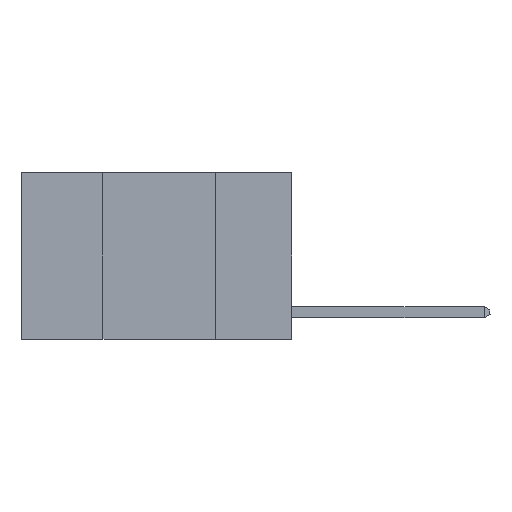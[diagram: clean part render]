
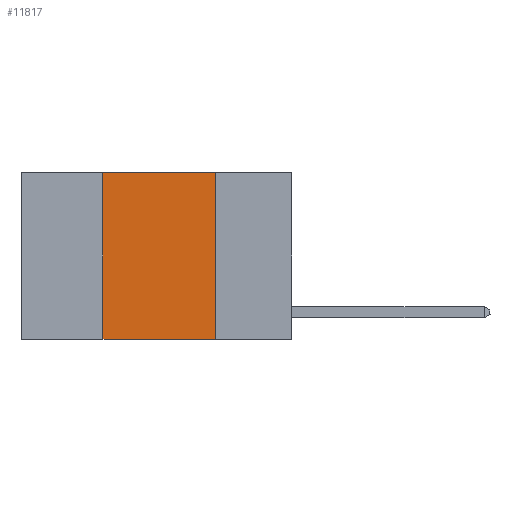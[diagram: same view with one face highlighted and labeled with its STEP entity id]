
A CAD part, left-side view. The second image highlights one B-rep face of the part: STEP entity #11817.
In plain terms, the highlighted planar face has unit normal (-1, 0, 0).
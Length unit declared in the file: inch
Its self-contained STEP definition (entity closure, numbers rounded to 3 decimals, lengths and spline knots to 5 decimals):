
#65 = VERTEX_POINT ( 'NONE', #8955 ) ;
#535 = LINE ( 'NONE', #18428, #4495 ) ;
#1374 = CARTESIAN_POINT ( 'NONE',  ( 0., 0.17, 0. ) ) ;
#2116 = EDGE_CURVE ( 'NONE', #18830, #6971, #5020, .T. ) ;
#3142 = DIRECTION ( 'NONE',  ( 0., 0., -1. ) ) ;
#4383 = EDGE_LOOP ( 'NONE', ( #15829, #8813, #13044, #15683 ) ) ;
#4392 = VECTOR ( 'NONE', #5676, 39.37008 ) ;
#4495 = VECTOR ( 'NONE', #13260, 39.37008 ) ;
#4566 = EDGE_CURVE ( 'NONE', #11226, #18830, #535, .T. ) ;
#4675 = AXIS2_PLACEMENT_3D ( 'NONE', #7570, #9560, #3142 ) ;
#5020 = LINE ( 'NONE', #12920, #7980 ) ;
#5676 = DIRECTION ( 'NONE',  ( 0., 0., -1. ) ) ;
#5678 = FACE_OUTER_BOUND ( 'NONE', #4383, .T. ) ;
#5888 = CARTESIAN_POINT ( 'NONE',  ( 0., 0.42, 0. ) ) ;
#6067 = VECTOR ( 'NONE', #16957, 39.37008 ) ;
#6500 = EDGE_CURVE ( 'NONE', #11226, #65, #10536, .T. ) ;
#6971 = VERTEX_POINT ( 'NONE', #1374 ) ;
#7246 = LINE ( 'NONE', #14931, #4392 ) ;
#7570 = CARTESIAN_POINT ( 'NONE',  ( 0., 0.6, 0. ) ) ;
#7980 = VECTOR ( 'NONE', #9772, 39.37008 ) ;
#8813 = ORIENTED_EDGE ( 'NONE', *, *, #2116, .F. ) ;
#8955 = CARTESIAN_POINT ( 'NONE',  ( 0., 0.17, -0.37 ) ) ;
#9560 = DIRECTION ( 'NONE',  ( 1., 0., 0. ) ) ;
#9772 = DIRECTION ( 'NONE',  ( 0., -1., 0. ) ) ;
#10536 = LINE ( 'NONE', #20039, #6067 ) ;
#11226 = VERTEX_POINT ( 'NONE', #12552 ) ;
#11817 = ADVANCED_FACE ( 'NONE', ( #5678 ), #15560, .F. ) ;
#12552 = CARTESIAN_POINT ( 'NONE',  ( 0., 0.42, -0.37 ) ) ;
#12920 = CARTESIAN_POINT ( 'NONE',  ( 0., 0.6, 0. ) ) ;
#13044 = ORIENTED_EDGE ( 'NONE', *, *, #4566, .F. ) ;
#13260 = DIRECTION ( 'NONE',  ( 0., 0., 1. ) ) ;
#14931 = CARTESIAN_POINT ( 'NONE',  ( 0., 0.17, 0. ) ) ;
#15560 = PLANE ( 'NONE',  #4675 ) ;
#15683 = ORIENTED_EDGE ( 'NONE', *, *, #6500, .T. ) ;
#15829 = ORIENTED_EDGE ( 'NONE', *, *, #15997, .F. ) ;
#15997 = EDGE_CURVE ( 'NONE', #6971, #65, #7246, .T. ) ;
#16957 = DIRECTION ( 'NONE',  ( 0., -1., 0. ) ) ;
#18428 = CARTESIAN_POINT ( 'NONE',  ( 0., 0.42, 0. ) ) ;
#18830 = VERTEX_POINT ( 'NONE', #5888 ) ;
#20039 = CARTESIAN_POINT ( 'NONE',  ( 0., 0.6, -0.37 ) ) ;
